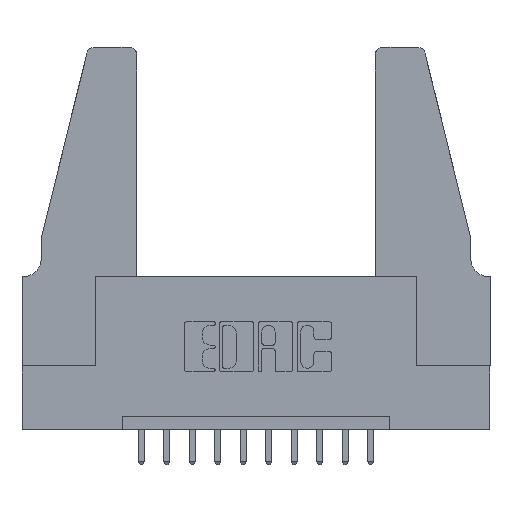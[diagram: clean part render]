
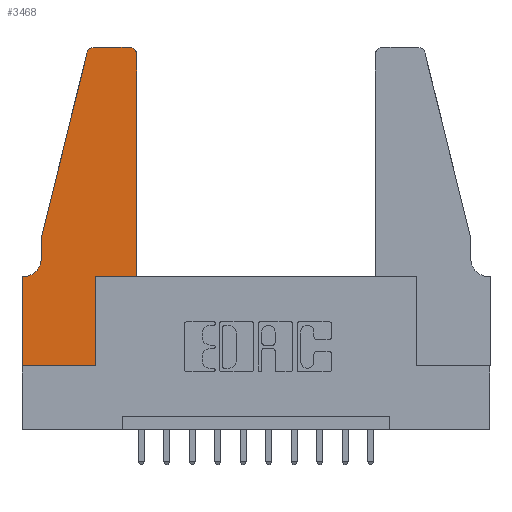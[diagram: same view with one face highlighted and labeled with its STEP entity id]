
A CAD part, top view. The second image highlights one B-rep face of the part: STEP entity #3468.
In plain terms, the highlighted planar face has unit normal (0, 0, 1).
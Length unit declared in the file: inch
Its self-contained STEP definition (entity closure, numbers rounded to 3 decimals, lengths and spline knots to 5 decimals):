
#278 = CIRCLE ( 'NONE', #2791, 0.03 ) ;
#308 = CARTESIAN_POINT ( 'NONE',  ( 0.4505, 0.35, 0.37 ) ) ;
#421 = LINE ( 'NONE', #7140, #1092 ) ;
#509 = EDGE_CURVE ( 'NONE', #9828, #13155, #11231, .T. ) ;
#657 = EDGE_LOOP ( 'NONE', ( #5002, #4049, #12870, #1812, #1744, #13415, #6886, #1349, #11774, #12567, #842, #1409 ) ) ;
#735 = CIRCLE ( 'NONE', #1902, 0.07 ) ;
#842 = ORIENTED_EDGE ( 'NONE', *, *, #509, .T. ) ;
#917 = DIRECTION ( 'NONE',  ( -1., 0., 0. ) ) ;
#998 = DIRECTION ( 'NONE',  ( 1., 0., 0. ) ) ;
#1092 = VECTOR ( 'NONE', #2512, 39.37008 ) ;
#1260 = FACE_OUTER_BOUND ( 'NONE', #657, .T. ) ;
#1279 = LINE ( 'NONE', #3278, #11484 ) ;
#1299 = LINE ( 'NONE', #11000, #11855 ) ;
#1349 = ORIENTED_EDGE ( 'NONE', *, *, #9695, .T. ) ;
#1366 = VERTEX_POINT ( 'NONE', #8963 ) ;
#1409 = ORIENTED_EDGE ( 'NONE', *, *, #3088, .T. ) ;
#1568 = DIRECTION ( 'NONE',  ( 0., 0., 1. ) ) ;
#1687 = VERTEX_POINT ( 'NONE', #12909 ) ;
#1717 = VERTEX_POINT ( 'NONE', #7663 ) ;
#1744 = ORIENTED_EDGE ( 'NONE', *, *, #6245, .T. ) ;
#1788 = CARTESIAN_POINT ( 'NONE',  ( 0.2865, 0.35, 0.37 ) ) ;
#1812 = ORIENTED_EDGE ( 'NONE', *, *, #11933, .T. ) ;
#1902 = AXIS2_PLACEMENT_3D ( 'NONE', #12968, #5433, #7592 ) ;
#2221 = VECTOR ( 'NONE', #7327, 39.37008 ) ;
#2512 = DIRECTION ( 'NONE',  ( 1., 0., 0. ) ) ;
#2791 = AXIS2_PLACEMENT_3D ( 'NONE', #7082, #1568, #8064 ) ;
#3088 = EDGE_CURVE ( 'NONE', #13155, #1366, #278, .T. ) ;
#3278 = CARTESIAN_POINT ( 'NONE',  ( 0.0755, 0.5, 0.37 ) ) ;
#3333 = VECTOR ( 'NONE', #917, 39.37008 ) ;
#3468 = ADVANCED_FACE ( 'NONE', ( #1260 ), #13406, .T. ) ;
#3889 = CARTESIAN_POINT ( 'NONE',  ( 0., 0., 0.37 ) ) ;
#4049 = ORIENTED_EDGE ( 'NONE', *, *, #9578, .T. ) ;
#4130 = CARTESIAN_POINT ( 'NONE',  ( 0.284, 1.25, 0.37 ) ) ;
#4535 = VERTEX_POINT ( 'NONE', #8232 ) ;
#4638 = DIRECTION ( 'NONE',  ( 0., -1., 0. ) ) ;
#4991 = LINE ( 'NONE', #13638, #2221 ) ;
#5002 = ORIENTED_EDGE ( 'NONE', *, *, #7114, .T. ) ;
#5039 = EDGE_CURVE ( 'NONE', #6973, #12485, #11303, .T. ) ;
#5433 = DIRECTION ( 'NONE',  ( 0., 0., -1. ) ) ;
#5543 = EDGE_CURVE ( 'NONE', #9521, #9828, #421, .T. ) ;
#5620 = AXIS2_PLACEMENT_3D ( 'NONE', #12384, #5660, #6752 ) ;
#5660 = DIRECTION ( 'NONE',  ( 0., 0., 1. ) ) ;
#5682 = CARTESIAN_POINT ( 'NONE',  ( 0.2865, 0.35, 0.37 ) ) ;
#5936 = AXIS2_PLACEMENT_3D ( 'NONE', #9037, #6916, #11158 ) ;
#6185 = VERTEX_POINT ( 'NONE', #11536 ) ;
#6245 = EDGE_CURVE ( 'NONE', #6185, #6973, #735, .T. ) ;
#6286 = LINE ( 'NONE', #3889, #9830 ) ;
#6752 = DIRECTION ( 'NONE',  ( 1., 0., 0. ) ) ;
#6763 = DIRECTION ( 'NONE',  ( -0.239, -0.971, 0. ) ) ;
#6886 = ORIENTED_EDGE ( 'NONE', *, *, #9923, .T. ) ;
#6916 = DIRECTION ( 'NONE',  ( 0., 0., 1. ) ) ;
#6973 = VERTEX_POINT ( 'NONE', #8302 ) ;
#7082 = CARTESIAN_POINT ( 'NONE',  ( 0.4205, 1.22, 0.37 ) ) ;
#7114 = EDGE_CURVE ( 'NONE', #1366, #13792, #4991, .T. ) ;
#7140 = CARTESIAN_POINT ( 'NONE',  ( 0.4505, 0.35, 0.37 ) ) ;
#7327 = DIRECTION ( 'NONE',  ( -1., 0., 0. ) ) ;
#7592 = DIRECTION ( 'NONE',  ( -1., 0., 0. ) ) ;
#7663 = CARTESIAN_POINT ( 'NONE',  ( 0., 0., 0.37 ) ) ;
#7797 = VERTEX_POINT ( 'NONE', #8946 ) ;
#8025 = EDGE_CURVE ( 'NONE', #4535, #9521, #10379, .T. ) ;
#8064 = DIRECTION ( 'NONE',  ( 1., 0., 0. ) ) ;
#8232 = CARTESIAN_POINT ( 'NONE',  ( 0.2865, 0., 0.37 ) ) ;
#8302 = CARTESIAN_POINT ( 'NONE',  ( 0.0055, 0.35, 0.37 ) ) ;
#8387 = DIRECTION ( 'NONE',  ( 0., 1., 0. ) ) ;
#8626 = CARTESIAN_POINT ( 'NONE',  ( 0.0755, 0.35, 0.37 ) ) ;
#8794 = LINE ( 'NONE', #10342, #12353 ) ;
#8946 = CARTESIAN_POINT ( 'NONE',  ( 0.25487, 1.22718, 0.37 ) ) ;
#8963 = CARTESIAN_POINT ( 'NONE',  ( 0.4205, 1.25, 0.37 ) ) ;
#9037 = CARTESIAN_POINT ( 'NONE',  ( 0., 0.35, 0.37 ) ) ;
#9222 = DIRECTION ( 'NONE',  ( 0., -1., 0. ) ) ;
#9521 = VERTEX_POINT ( 'NONE', #5682 ) ;
#9578 = EDGE_CURVE ( 'NONE', #13792, #7797, #11362, .T. ) ;
#9616 = CARTESIAN_POINT ( 'NONE',  ( 0.4505, 0.35, 0.37 ) ) ;
#9695 = EDGE_CURVE ( 'NONE', #1717, #4535, #6286, .T. ) ;
#9828 = VERTEX_POINT ( 'NONE', #9616 ) ;
#9830 = VECTOR ( 'NONE', #998, 39.37008 ) ;
#9923 = EDGE_CURVE ( 'NONE', #12485, #1717, #1299, .T. ) ;
#10342 = CARTESIAN_POINT ( 'NONE',  ( 0.0755, 0.5, 0.37 ) ) ;
#10371 = CARTESIAN_POINT ( 'NONE',  ( 0.4505, 1.22, 0.37 ) ) ;
#10379 = LINE ( 'NONE', #1788, #12565 ) ;
#10388 = CARTESIAN_POINT ( 'NONE',  ( 0., 0.35, 0.37 ) ) ;
#11000 = CARTESIAN_POINT ( 'NONE',  ( 0., 0., 0.37 ) ) ;
#11158 = DIRECTION ( 'NONE',  ( 1., 0., 0. ) ) ;
#11231 = LINE ( 'NONE', #308, #11749 ) ;
#11303 = LINE ( 'NONE', #8626, #3333 ) ;
#11362 = CIRCLE ( 'NONE', #5620, 0.03 ) ;
#11484 = VECTOR ( 'NONE', #6763, 39.37008 ) ;
#11536 = CARTESIAN_POINT ( 'NONE',  ( 0.0755, 0.42, 0.37 ) ) ;
#11749 = VECTOR ( 'NONE', #12116, 39.37008 ) ;
#11774 = ORIENTED_EDGE ( 'NONE', *, *, #8025, .T. ) ;
#11855 = VECTOR ( 'NONE', #4638, 39.37008 ) ;
#11933 = EDGE_CURVE ( 'NONE', #1687, #6185, #8794, .T. ) ;
#12116 = DIRECTION ( 'NONE',  ( 0., 1., 0. ) ) ;
#12353 = VECTOR ( 'NONE', #9222, 39.37008 ) ;
#12384 = CARTESIAN_POINT ( 'NONE',  ( 0.284, 1.22, 0.37 ) ) ;
#12485 = VERTEX_POINT ( 'NONE', #10388 ) ;
#12565 = VECTOR ( 'NONE', #8387, 39.37008 ) ;
#12567 = ORIENTED_EDGE ( 'NONE', *, *, #5543, .T. ) ;
#12819 = EDGE_CURVE ( 'NONE', #7797, #1687, #1279, .T. ) ;
#12870 = ORIENTED_EDGE ( 'NONE', *, *, #12819, .T. ) ;
#12909 = CARTESIAN_POINT ( 'NONE',  ( 0.0755, 0.5, 0.37 ) ) ;
#12968 = CARTESIAN_POINT ( 'NONE',  ( 0.0055, 0.42, 0.37 ) ) ;
#13155 = VERTEX_POINT ( 'NONE', #10371 ) ;
#13406 = PLANE ( 'NONE',  #5936 ) ;
#13415 = ORIENTED_EDGE ( 'NONE', *, *, #5039, .T. ) ;
#13638 = CARTESIAN_POINT ( 'NONE',  ( 0.2605, 1.25, 0.37 ) ) ;
#13792 = VERTEX_POINT ( 'NONE', #4130 ) ;
